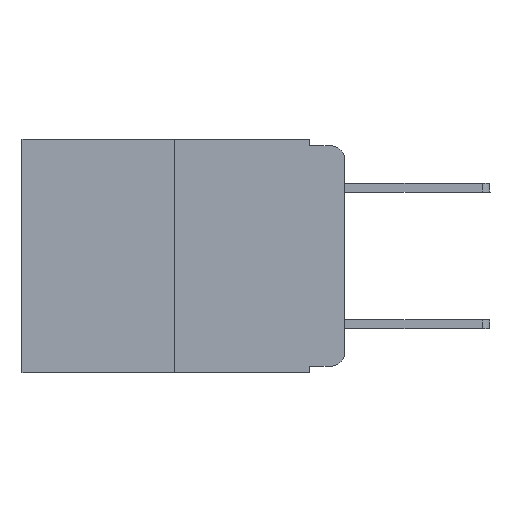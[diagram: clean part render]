
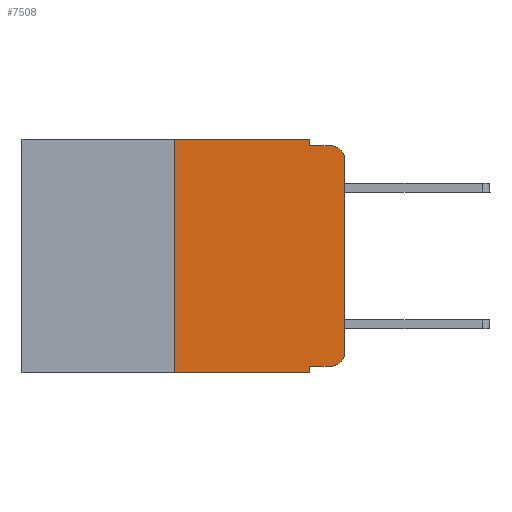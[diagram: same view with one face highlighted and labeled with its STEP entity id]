
A CAD part, left-side view. The second image highlights one B-rep face of the part: STEP entity #7508.
In plain terms, the highlighted planar face has unit normal (-1, 0, 0).
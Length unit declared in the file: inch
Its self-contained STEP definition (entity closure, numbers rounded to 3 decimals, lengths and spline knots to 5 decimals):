
#31 = ORIENTED_EDGE ( 'NONE', *, *, #3542, .F. ) ;
#113 = AXIS2_PLACEMENT_3D ( 'NONE', #2230, #7497, #5285 ) ;
#195 = CARTESIAN_POINT ( 'NONE',  ( 0., 0.051, -0.01 ) ) ;
#222 = ORIENTED_EDGE ( 'NONE', *, *, #8455, .T. ) ;
#276 = VERTEX_POINT ( 'NONE', #9643 ) ;
#357 = VERTEX_POINT ( 'NONE', #8103 ) ;
#392 = VECTOR ( 'NONE', #3219, 39.37008 ) ;
#558 = VERTEX_POINT ( 'NONE', #4616 ) ;
#587 = VECTOR ( 'NONE', #943, 39.37008 ) ;
#939 = ORIENTED_EDGE ( 'NONE', *, *, #944, .T. ) ;
#943 = DIRECTION ( 'NONE',  ( 0., 0., -1. ) ) ;
#944 = EDGE_CURVE ( 'NONE', #1400, #558, #6232, .T. ) ;
#956 = VECTOR ( 'NONE', #4377, 39.37008 ) ;
#995 = CARTESIAN_POINT ( 'NONE',  ( 0., 0.02, -0.01 ) ) ;
#1129 = CARTESIAN_POINT ( 'NONE',  ( 0., 0.25, -0.343 ) ) ;
#1296 = LINE ( 'NONE', #1573, #1532 ) ;
#1324 = VERTEX_POINT ( 'NONE', #3842 ) ;
#1343 = VECTOR ( 'NONE', #4750, 39.37008 ) ;
#1400 = VERTEX_POINT ( 'NONE', #5221 ) ;
#1532 = VECTOR ( 'NONE', #4534, 39.37008 ) ;
#1573 = CARTESIAN_POINT ( 'NONE',  ( 0., 0.25, 0. ) ) ;
#1675 = VECTOR ( 'NONE', #7578, 39.37008 ) ;
#1776 = EDGE_LOOP ( 'NONE', ( #3040, #3643, #2934, #5386, #9507, #31, #9130, #2053, #939, #222 ) ) ;
#2053 = ORIENTED_EDGE ( 'NONE', *, *, #3345, .F. ) ;
#2230 = CARTESIAN_POINT ( 'NONE',  ( 0., 0.02, -0.313 ) ) ;
#2562 = VERTEX_POINT ( 'NONE', #3267 ) ;
#2631 = LINE ( 'NONE', #3916, #1343 ) ;
#2806 = EDGE_CURVE ( 'NONE', #9427, #357, #3781, .T. ) ;
#2934 = ORIENTED_EDGE ( 'NONE', *, *, #6670, .F. ) ;
#3040 = ORIENTED_EDGE ( 'NONE', *, *, #4329, .T. ) ;
#3219 = DIRECTION ( 'NONE',  ( 0., -1., 0. ) ) ;
#3267 = CARTESIAN_POINT ( 'NONE',  ( 0., 0.051, -0.01 ) ) ;
#3345 = EDGE_CURVE ( 'NONE', #1400, #357, #3771, .T. ) ;
#3451 = CARTESIAN_POINT ( 'NONE',  ( 0., 0.25, 0. ) ) ;
#3456 = VECTOR ( 'NONE', #5122, 39.37008 ) ;
#3542 = EDGE_CURVE ( 'NONE', #9427, #8183, #1296, .T. ) ;
#3643 = ORIENTED_EDGE ( 'NONE', *, *, #9154, .T. ) ;
#3771 = LINE ( 'NONE', #4731, #587 ) ;
#3781 = LINE ( 'NONE', #6674, #956 ) ;
#3842 = CARTESIAN_POINT ( 'NONE',  ( 0., 0., -0.03 ) ) ;
#3916 = CARTESIAN_POINT ( 'NONE',  ( 0., 0., 0. ) ) ;
#4257 = VERTEX_POINT ( 'NONE', #995 ) ;
#4329 = EDGE_CURVE ( 'NONE', #276, #1324, #2631, .T. ) ;
#4377 = DIRECTION ( 'NONE',  ( 0., -1., 0. ) ) ;
#4399 = VECTOR ( 'NONE', #6495, 39.37008 ) ;
#4534 = DIRECTION ( 'NONE',  ( 0., 0., 1. ) ) ;
#4616 = CARTESIAN_POINT ( 'NONE',  ( 0., 0.02, -0.333 ) ) ;
#4645 = EDGE_CURVE ( 'NONE', #8183, #7444, #4999, .T. ) ;
#4715 = FACE_OUTER_BOUND ( 'NONE', #1776, .T. ) ;
#4731 = CARTESIAN_POINT ( 'NONE',  ( 0., 0.051, 0. ) ) ;
#4750 = DIRECTION ( 'NONE',  ( 0., 0., 1. ) ) ;
#4977 = LINE ( 'NONE', #195, #392 ) ;
#4999 = LINE ( 'NONE', #8094, #3456 ) ;
#5040 = CARTESIAN_POINT ( 'NONE',  ( 0., 0.051, -0.333 ) ) ;
#5122 = DIRECTION ( 'NONE',  ( 0., -1., 0. ) ) ;
#5221 = CARTESIAN_POINT ( 'NONE',  ( 0., 0.051, -0.333 ) ) ;
#5285 = DIRECTION ( 'NONE',  ( 0., 0., -1. ) ) ;
#5309 = CARTESIAN_POINT ( 'NONE',  ( 0., 0.02, -0.03 ) ) ;
#5386 = ORIENTED_EDGE ( 'NONE', *, *, #6064, .F. ) ;
#5478 = DIRECTION ( 'NONE',  ( 1., 0., 0. ) ) ;
#6064 = EDGE_CURVE ( 'NONE', #7444, #2562, #7248, .T. ) ;
#6232 = LINE ( 'NONE', #5040, #4399 ) ;
#6291 = PLANE ( 'NONE',  #9132 ) ;
#6495 = DIRECTION ( 'NONE',  ( 0., -1., 0. ) ) ;
#6670 = EDGE_CURVE ( 'NONE', #2562, #4257, #4977, .T. ) ;
#6674 = CARTESIAN_POINT ( 'NONE',  ( 0., 0.473, -0.343 ) ) ;
#6815 = CARTESIAN_POINT ( 'NONE',  ( 0., 0.051, 0. ) ) ;
#7248 = LINE ( 'NONE', #6815, #1675 ) ;
#7444 = VERTEX_POINT ( 'NONE', #8408 ) ;
#7497 = DIRECTION ( 'NONE',  ( -1., 0., 0. ) ) ;
#7508 = ADVANCED_FACE ( 'NONE', ( #4715 ), #6291, .F. ) ;
#7578 = DIRECTION ( 'NONE',  ( 0., 0., -1. ) ) ;
#7649 = CIRCLE ( 'NONE', #9703, 0.02 ) ;
#7750 = CARTESIAN_POINT ( 'NONE',  ( 0., 0.473, 0. ) ) ;
#8094 = CARTESIAN_POINT ( 'NONE',  ( 0., 0.473, 0. ) ) ;
#8103 = CARTESIAN_POINT ( 'NONE',  ( 0., 0.051, -0.343 ) ) ;
#8183 = VERTEX_POINT ( 'NONE', #3451 ) ;
#8260 = CIRCLE ( 'NONE', #113, 0.02 ) ;
#8408 = CARTESIAN_POINT ( 'NONE',  ( 0., 0.051, 0. ) ) ;
#8455 = EDGE_CURVE ( 'NONE', #558, #276, #8260, .T. ) ;
#8511 = DIRECTION ( 'NONE',  ( 0., 0., -1. ) ) ;
#8998 = DIRECTION ( 'NONE',  ( 0., 0., -1. ) ) ;
#9099 = DIRECTION ( 'NONE',  ( -1., 0., 0. ) ) ;
#9130 = ORIENTED_EDGE ( 'NONE', *, *, #2806, .T. ) ;
#9132 = AXIS2_PLACEMENT_3D ( 'NONE', #7750, #5478, #8511 ) ;
#9154 = EDGE_CURVE ( 'NONE', #1324, #4257, #7649, .T. ) ;
#9427 = VERTEX_POINT ( 'NONE', #1129 ) ;
#9507 = ORIENTED_EDGE ( 'NONE', *, *, #4645, .F. ) ;
#9643 = CARTESIAN_POINT ( 'NONE',  ( 0., 0., -0.313 ) ) ;
#9703 = AXIS2_PLACEMENT_3D ( 'NONE', #5309, #9099, #8998 ) ;
